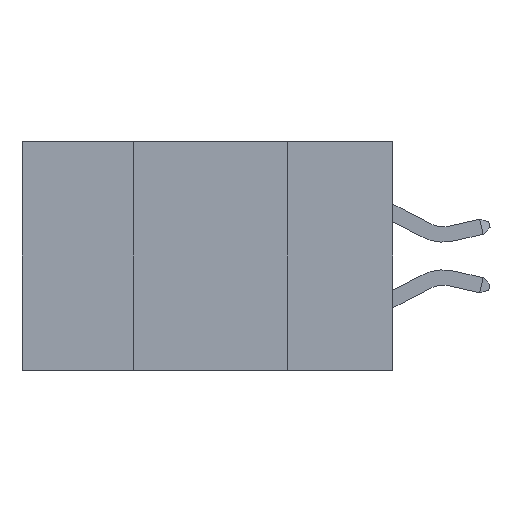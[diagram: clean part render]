
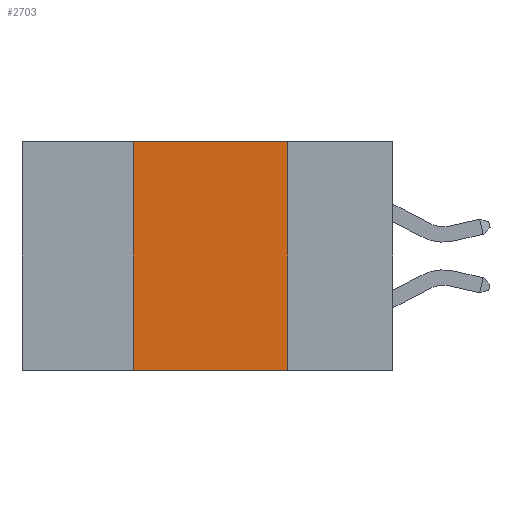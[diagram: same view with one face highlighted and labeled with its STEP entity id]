
A CAD part, left-side view. The second image highlights one B-rep face of the part: STEP entity #2703.
In plain terms, the highlighted planar face has unit normal (-1, 0, 0).
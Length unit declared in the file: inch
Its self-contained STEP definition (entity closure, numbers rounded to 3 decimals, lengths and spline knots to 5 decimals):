
#508 = DIRECTION ( 'NONE',  ( 0., 0., -1. ) ) ;
#571 = PLANE ( 'NONE',  #5781 ) ;
#1259 = CARTESIAN_POINT ( 'NONE',  ( 0., 0.6, -0.37 ) ) ;
#2703 = ADVANCED_FACE ( 'NONE', ( #12255 ), #571, .F. ) ;
#2988 = VECTOR ( 'NONE', #14992, 39.37008 ) ;
#3244 = VERTEX_POINT ( 'NONE', #9931 ) ;
#4168 = VERTEX_POINT ( 'NONE', #13082 ) ;
#4271 = ORIENTED_EDGE ( 'NONE', *, *, #7012, .F. ) ;
#4416 = ORIENTED_EDGE ( 'NONE', *, *, #13378, .F. ) ;
#5781 = AXIS2_PLACEMENT_3D ( 'NONE', #8278, #9632, #508 ) ;
#5943 = DIRECTION ( 'NONE',  ( 0., -1., 0. ) ) ;
#6774 = LINE ( 'NONE', #11136, #17509 ) ;
#7012 = EDGE_CURVE ( 'NONE', #3244, #15627, #6774, .T. ) ;
#8278 = CARTESIAN_POINT ( 'NONE',  ( 0., 0.6, 0. ) ) ;
#8934 = LINE ( 'NONE', #13939, #17717 ) ;
#9632 = DIRECTION ( 'NONE',  ( 1., 0., 0. ) ) ;
#9931 = CARTESIAN_POINT ( 'NONE',  ( 0., 0.42, 0. ) ) ;
#10187 = ORIENTED_EDGE ( 'NONE', *, *, #15751, .F. ) ;
#10894 = CARTESIAN_POINT ( 'NONE',  ( 0., 0.42, -0.37 ) ) ;
#10996 = EDGE_LOOP ( 'NONE', ( #10187, #4271, #4416, #13384 ) ) ;
#10997 = CARTESIAN_POINT ( 'NONE',  ( 0., 0.17, 0. ) ) ;
#11136 = CARTESIAN_POINT ( 'NONE',  ( 0., 0.6, 0. ) ) ;
#11469 = DIRECTION ( 'NONE',  ( 0., 0., 1. ) ) ;
#12255 = FACE_OUTER_BOUND ( 'NONE', #10996, .T. ) ;
#13082 = CARTESIAN_POINT ( 'NONE',  ( 0., 0.17, -0.37 ) ) ;
#13150 = CARTESIAN_POINT ( 'NONE',  ( 0., 0.42, 0. ) ) ;
#13378 = EDGE_CURVE ( 'NONE', #17758, #3244, #18913, .T. ) ;
#13384 = ORIENTED_EDGE ( 'NONE', *, *, #13647, .T. ) ;
#13647 = EDGE_CURVE ( 'NONE', #17758, #4168, #16777, .T. ) ;
#13939 = CARTESIAN_POINT ( 'NONE',  ( 0., 0.17, 0. ) ) ;
#14992 = DIRECTION ( 'NONE',  ( 0., -1., 0. ) ) ;
#15444 = DIRECTION ( 'NONE',  ( 0., 0., -1. ) ) ;
#15627 = VERTEX_POINT ( 'NONE', #10997 ) ;
#15751 = EDGE_CURVE ( 'NONE', #15627, #4168, #8934, .T. ) ;
#16777 = LINE ( 'NONE', #1259, #2988 ) ;
#17509 = VECTOR ( 'NONE', #5943, 39.37008 ) ;
#17717 = VECTOR ( 'NONE', #15444, 39.37008 ) ;
#17758 = VERTEX_POINT ( 'NONE', #10894 ) ;
#18913 = LINE ( 'NONE', #13150, #19128 ) ;
#19128 = VECTOR ( 'NONE', #11469, 39.37008 ) ;
